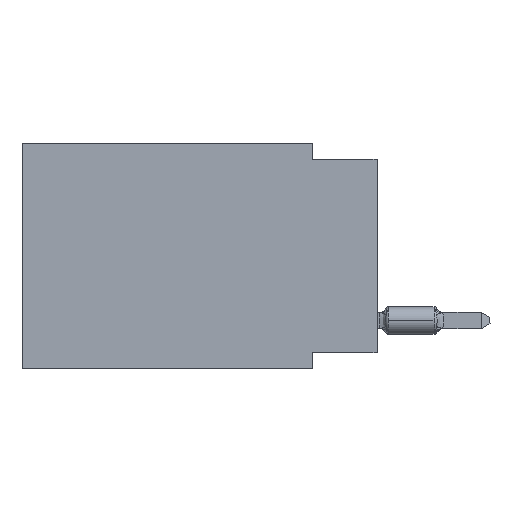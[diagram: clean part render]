
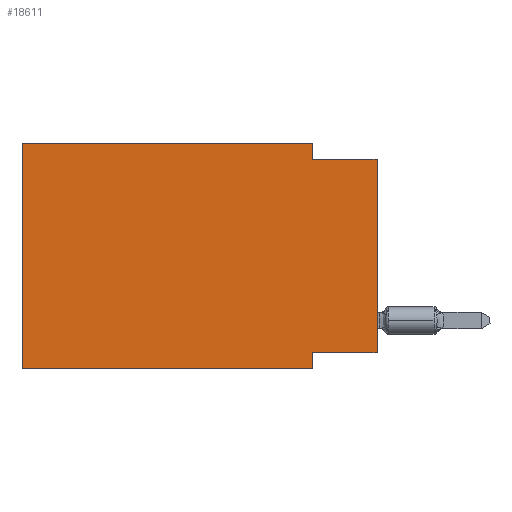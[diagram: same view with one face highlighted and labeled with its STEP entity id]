
A CAD part, left-side view. The second image highlights one B-rep face of the part: STEP entity #18611.
In plain terms, the highlighted planar face has unit normal (-1, 0, 0).
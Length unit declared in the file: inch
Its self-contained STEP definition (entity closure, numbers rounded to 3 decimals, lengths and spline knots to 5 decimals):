
#347 = VERTEX_POINT ( 'NONE', #17684 ) ;
#626 = EDGE_CURVE ( 'NONE', #1360, #2205, #11694, .T. ) ;
#668 = CARTESIAN_POINT ( 'NONE',  ( 0., 0., -0.025 ) ) ;
#997 = LINE ( 'NONE', #6292, #4798 ) ;
#1159 = VERTEX_POINT ( 'NONE', #3640 ) ;
#1198 = VERTEX_POINT ( 'NONE', #16616 ) ;
#1360 = VERTEX_POINT ( 'NONE', #15524 ) ;
#2205 = VERTEX_POINT ( 'NONE', #14756 ) ;
#3144 = EDGE_CURVE ( 'NONE', #15732, #1360, #997, .T. ) ;
#3352 = ORIENTED_EDGE ( 'NONE', *, *, #17733, .T. ) ;
#3411 = ORIENTED_EDGE ( 'NONE', *, *, #10258, .F. ) ;
#3456 = EDGE_LOOP ( 'NONE', ( #5483, #13433, #13410, #7226, #10496, #3352, #5711, #3411 ) ) ;
#3640 = CARTESIAN_POINT ( 'NONE',  ( 0., 0.1, -0.35 ) ) ;
#3891 = VECTOR ( 'NONE', #6022, 39.37008 ) ;
#4450 = EDGE_CURVE ( 'NONE', #1198, #2205, #8564, .T. ) ;
#4798 = VECTOR ( 'NONE', #11169, 39.37008 ) ;
#5063 = LINE ( 'NONE', #7714, #13163 ) ;
#5113 = VECTOR ( 'NONE', #5917, 39.37008 ) ;
#5202 = FACE_OUTER_BOUND ( 'NONE', #3456, .T. ) ;
#5483 = ORIENTED_EDGE ( 'NONE', *, *, #4450, .T. ) ;
#5711 = ORIENTED_EDGE ( 'NONE', *, *, #13628, .F. ) ;
#5917 = DIRECTION ( 'NONE',  ( 0., 0., -1. ) ) ;
#6022 = DIRECTION ( 'NONE',  ( 0., 0., 1. ) ) ;
#6292 = CARTESIAN_POINT ( 'NONE',  ( 0., 0.1, 0. ) ) ;
#6879 = CARTESIAN_POINT ( 'NONE',  ( 0., 0.55, 0. ) ) ;
#6950 = DIRECTION ( 'NONE',  ( 1., 0., 0. ) ) ;
#6975 = DIRECTION ( 'NONE',  ( 0., 1., 0. ) ) ;
#7226 = ORIENTED_EDGE ( 'NONE', *, *, #15029, .F. ) ;
#7417 = VECTOR ( 'NONE', #16842, 39.37008 ) ;
#7574 = CARTESIAN_POINT ( 'NONE',  ( 0., 0.1, -0.35 ) ) ;
#7714 = CARTESIAN_POINT ( 'NONE',  ( 0., 0.55, 0. ) ) ;
#8044 = CARTESIAN_POINT ( 'NONE',  ( 0., 0.1, 0. ) ) ;
#8564 = LINE ( 'NONE', #18662, #9570 ) ;
#8703 = VERTEX_POINT ( 'NONE', #15982 ) ;
#8711 = LINE ( 'NONE', #17285, #3891 ) ;
#9055 = DIRECTION ( 'NONE',  ( 0., 0., 1. ) ) ;
#9369 = DIRECTION ( 'NONE',  ( 0., -1., 0. ) ) ;
#9570 = VECTOR ( 'NONE', #9055, 39.37008 ) ;
#10258 = EDGE_CURVE ( 'NONE', #1198, #347, #20859, .T. ) ;
#10496 = ORIENTED_EDGE ( 'NONE', *, *, #13036, .F. ) ;
#11169 = DIRECTION ( 'NONE',  ( 0., 0., -1. ) ) ;
#11500 = VECTOR ( 'NONE', #20448, 39.37008 ) ;
#11694 = LINE ( 'NONE', #668, #7417 ) ;
#12502 = CARTESIAN_POINT ( 'NONE',  ( 0., 0.55, -0.35 ) ) ;
#13036 = EDGE_CURVE ( 'NONE', #8703, #16571, #8711, .T. ) ;
#13163 = VECTOR ( 'NONE', #9369, 39.37008 ) ;
#13410 = ORIENTED_EDGE ( 'NONE', *, *, #3144, .F. ) ;
#13433 = ORIENTED_EDGE ( 'NONE', *, *, #626, .F. ) ;
#13628 = EDGE_CURVE ( 'NONE', #347, #1159, #17954, .T. ) ;
#14756 = CARTESIAN_POINT ( 'NONE',  ( 0., 0., -0.025 ) ) ;
#15026 = PLANE ( 'NONE',  #16562 ) ;
#15029 = EDGE_CURVE ( 'NONE', #16571, #15732, #5063, .T. ) ;
#15049 = CARTESIAN_POINT ( 'NONE',  ( 0., 0., -0.325 ) ) ;
#15524 = CARTESIAN_POINT ( 'NONE',  ( 0., 0.1, -0.025 ) ) ;
#15732 = VERTEX_POINT ( 'NONE', #8044 ) ;
#15817 = LINE ( 'NONE', #12502, #11500 ) ;
#15982 = CARTESIAN_POINT ( 'NONE',  ( 0., 0.55, -0.35 ) ) ;
#16562 = AXIS2_PLACEMENT_3D ( 'NONE', #6879, #6950, #18192 ) ;
#16571 = VERTEX_POINT ( 'NONE', #18537 ) ;
#16616 = CARTESIAN_POINT ( 'NONE',  ( 0., 0., -0.325 ) ) ;
#16645 = VECTOR ( 'NONE', #6975, 39.37008 ) ;
#16842 = DIRECTION ( 'NONE',  ( 0., -1., 0. ) ) ;
#17285 = CARTESIAN_POINT ( 'NONE',  ( 0., 0.55, 0. ) ) ;
#17684 = CARTESIAN_POINT ( 'NONE',  ( 0., 0.1, -0.325 ) ) ;
#17733 = EDGE_CURVE ( 'NONE', #8703, #1159, #15817, .T. ) ;
#17954 = LINE ( 'NONE', #7574, #5113 ) ;
#18192 = DIRECTION ( 'NONE',  ( 0., 0., -1. ) ) ;
#18537 = CARTESIAN_POINT ( 'NONE',  ( 0., 0.55, 0. ) ) ;
#18611 = ADVANCED_FACE ( 'NONE', ( #5202 ), #15026, .F. ) ;
#18662 = CARTESIAN_POINT ( 'NONE',  ( 0., 0., 0. ) ) ;
#20448 = DIRECTION ( 'NONE',  ( 0., -1., 0. ) ) ;
#20859 = LINE ( 'NONE', #15049, #16645 ) ;
